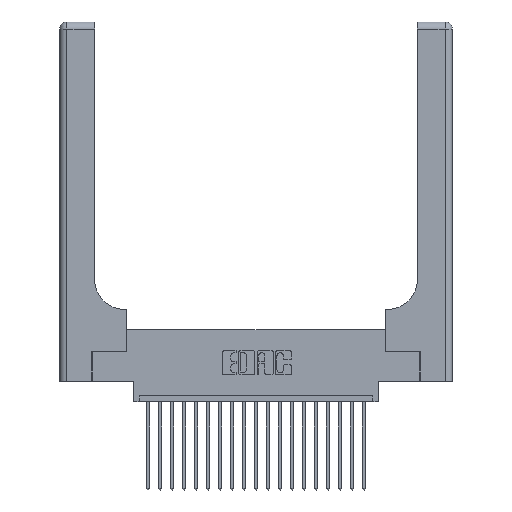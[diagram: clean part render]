
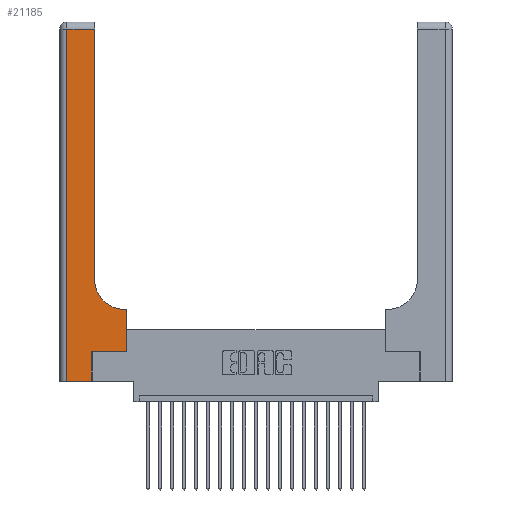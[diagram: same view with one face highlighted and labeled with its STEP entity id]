
A CAD part, top view. The second image highlights one B-rep face of the part: STEP entity #21185.
In plain terms, the highlighted planar face has unit normal (0, 0, 1).
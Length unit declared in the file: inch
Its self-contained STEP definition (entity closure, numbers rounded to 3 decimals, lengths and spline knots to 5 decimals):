
#96 = VERTEX_POINT ( 'NONE', #8171 ) ;
#710 = PLANE ( 'NONE',  #10663 ) ;
#1420 = LINE ( 'NONE', #10987, #13202 ) ;
#1552 = CARTESIAN_POINT ( 'NONE',  ( 0.06, 0., 0.37 ) ) ;
#1995 = CARTESIAN_POINT ( 'NONE',  ( 0., 2.94, 0.37 ) ) ;
#2049 = LINE ( 'NONE', #7131, #10278 ) ;
#2213 = EDGE_CURVE ( 'NONE', #11466, #96, #12198, .T. ) ;
#2623 = DIRECTION ( 'NONE',  ( -1., 0., 0. ) ) ;
#2770 = CARTESIAN_POINT ( 'NONE',  ( 0.06, 3., 0.37 ) ) ;
#2963 = LINE ( 'NONE', #9345, #3492 ) ;
#3492 = VECTOR ( 'NONE', #15045, 39.37008 ) ;
#3724 = ORIENTED_EDGE ( 'NONE', *, *, #8229, .T. ) ;
#3832 = VERTEX_POINT ( 'NONE', #10548 ) ;
#4297 = EDGE_CURVE ( 'NONE', #96, #5940, #20085, .T. ) ;
#4305 = VECTOR ( 'NONE', #5833, 39.37008 ) ;
#5180 = DIRECTION ( 'NONE',  ( 0., 1., 0. ) ) ;
#5833 = DIRECTION ( 'NONE',  ( -1., 0., 0. ) ) ;
#5940 = VERTEX_POINT ( 'NONE', #21652 ) ;
#6116 = CARTESIAN_POINT ( 'NONE',  ( 0., 3., 0.37 ) ) ;
#6199 = CARTESIAN_POINT ( 'NONE',  ( 0.5585, 0.25, 0.37 ) ) ;
#6351 = VERTEX_POINT ( 'NONE', #12608 ) ;
#6671 = VECTOR ( 'NONE', #5180, 39.37008 ) ;
#6928 = VERTEX_POINT ( 'NONE', #1552 ) ;
#7041 = DIRECTION ( 'NONE',  ( 1., 0., 0. ) ) ;
#7126 = EDGE_LOOP ( 'NONE', ( #14949, #3724, #7779, #18496, #15328, #12062, #15010, #16001, #8026 ) ) ;
#7131 = CARTESIAN_POINT ( 'NONE',  ( 0.269, 0.25, 0.37 ) ) ;
#7281 = LINE ( 'NONE', #1995, #4305 ) ;
#7779 = ORIENTED_EDGE ( 'NONE', *, *, #8827, .T. ) ;
#8026 = ORIENTED_EDGE ( 'NONE', *, *, #13165, .T. ) ;
#8171 = CARTESIAN_POINT ( 'NONE',  ( 0.5585, 0.6, 0.37 ) ) ;
#8229 = EDGE_CURVE ( 'NONE', #9299, #6351, #7281, .T. ) ;
#8827 = EDGE_CURVE ( 'NONE', #6351, #6928, #9760, .T. ) ;
#8890 = CARTESIAN_POINT ( 'NONE',  ( 0.2915, 3., 0.37 ) ) ;
#9009 = EDGE_CURVE ( 'NONE', #3832, #9299, #22659, .T. ) ;
#9053 = CARTESIAN_POINT ( 'NONE',  ( 0.5415, 0.85, 0.37 ) ) ;
#9204 = VERTEX_POINT ( 'NONE', #18484 ) ;
#9299 = VERTEX_POINT ( 'NONE', #11941 ) ;
#9345 = CARTESIAN_POINT ( 'NONE',  ( 0.269, 0., 0.37 ) ) ;
#9469 = VECTOR ( 'NONE', #19402, 39.37008 ) ;
#9760 = LINE ( 'NONE', #2770, #15809 ) ;
#9882 = VECTOR ( 'NONE', #12719, 39.37008 ) ;
#10210 = CARTESIAN_POINT ( 'NONE',  ( 0.269, 0.25, 0.37 ) ) ;
#10278 = VECTOR ( 'NONE', #16075, 39.37008 ) ;
#10548 = CARTESIAN_POINT ( 'NONE',  ( 0.2915, 0.85, 0.37 ) ) ;
#10663 = AXIS2_PLACEMENT_3D ( 'NONE', #6116, #14820, #2623 ) ;
#10987 = CARTESIAN_POINT ( 'NONE',  ( 0., 0., 0.37 ) ) ;
#11338 = EDGE_CURVE ( 'NONE', #6928, #9204, #1420, .T. ) ;
#11466 = VERTEX_POINT ( 'NONE', #12444 ) ;
#11889 = DIRECTION ( 'NONE',  ( 0., -1., 0. ) ) ;
#11941 = CARTESIAN_POINT ( 'NONE',  ( 0.2915, 2.94, 0.37 ) ) ;
#12062 = ORIENTED_EDGE ( 'NONE', *, *, #12669, .T. ) ;
#12198 = LINE ( 'NONE', #6199, #6671 ) ;
#12444 = CARTESIAN_POINT ( 'NONE',  ( 0.5585, 0.25, 0.37 ) ) ;
#12608 = CARTESIAN_POINT ( 'NONE',  ( 0.06, 2.94, 0.37 ) ) ;
#12669 = EDGE_CURVE ( 'NONE', #14548, #11466, #2049, .T. ) ;
#12719 = DIRECTION ( 'NONE',  ( -1., 0., 0. ) ) ;
#13165 = EDGE_CURVE ( 'NONE', #5940, #3832, #21807, .T. ) ;
#13202 = VECTOR ( 'NONE', #14425, 39.37008 ) ;
#14230 = AXIS2_PLACEMENT_3D ( 'NONE', #9053, #15629, #7041 ) ;
#14425 = DIRECTION ( 'NONE',  ( 1., 0., 0. ) ) ;
#14548 = VERTEX_POINT ( 'NONE', #10210 ) ;
#14820 = DIRECTION ( 'NONE',  ( 0., 0., -1. ) ) ;
#14949 = ORIENTED_EDGE ( 'NONE', *, *, #9009, .T. ) ;
#15010 = ORIENTED_EDGE ( 'NONE', *, *, #2213, .T. ) ;
#15045 = DIRECTION ( 'NONE',  ( 0., 1., 0. ) ) ;
#15328 = ORIENTED_EDGE ( 'NONE', *, *, #21162, .T. ) ;
#15629 = DIRECTION ( 'NONE',  ( 0., 0., -1. ) ) ;
#15809 = VECTOR ( 'NONE', #11889, 39.37008 ) ;
#16001 = ORIENTED_EDGE ( 'NONE', *, *, #4297, .T. ) ;
#16075 = DIRECTION ( 'NONE',  ( 1., 0., 0. ) ) ;
#18117 = CARTESIAN_POINT ( 'NONE',  ( 0.2915, 0.6, 0.37 ) ) ;
#18484 = CARTESIAN_POINT ( 'NONE',  ( 0.269, 0., 0.37 ) ) ;
#18496 = ORIENTED_EDGE ( 'NONE', *, *, #11338, .T. ) ;
#18931 = FACE_OUTER_BOUND ( 'NONE', #7126, .T. ) ;
#19402 = DIRECTION ( 'NONE',  ( 0., 1., 0. ) ) ;
#20085 = LINE ( 'NONE', #18117, #9882 ) ;
#21162 = EDGE_CURVE ( 'NONE', #9204, #14548, #2963, .T. ) ;
#21185 = ADVANCED_FACE ( 'NONE', ( #18931 ), #710, .F. ) ;
#21652 = CARTESIAN_POINT ( 'NONE',  ( 0.5415, 0.6, 0.37 ) ) ;
#21807 = CIRCLE ( 'NONE', #14230, 0.25 ) ;
#22659 = LINE ( 'NONE', #8890, #9469 ) ;
